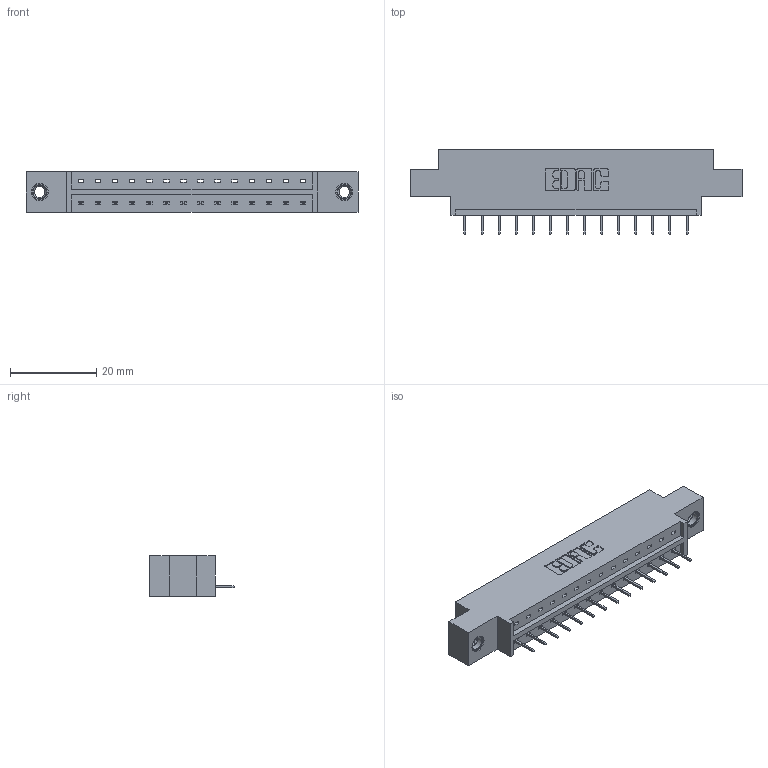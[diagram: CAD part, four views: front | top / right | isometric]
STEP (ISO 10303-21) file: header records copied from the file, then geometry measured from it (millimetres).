
FILE_DESCRIPTION (( 'STEP AP203' ), '1' );
FILE_NAME ('333-014-524-607.STEP', '2018-08-01T02:20:03', ( '' ), ( '' ), 'SwSTEP 2.0', 'SolidWorks 2016', '' );
FILE_SCHEMA (( 'CONFIG_CONTROL_DESIGN' ));
Length unit declared in the file: inch
Products named in the file (4): 333 Part_Offset - .156 Dia - TI; 345-292-001_345-293-124; 345-250-001_345-250-005-103; 333-014-524-607
Assembly tree (17 placements, depth 2):
  333-014-524-607
    333 Part_Offset - .156 Dia - TI
    345-292-001_345-293-124  x14
    345-250-001_345-250-005-103  x2
Bounding box: 77.01 x 19.69 x 9.4 mm (x, y, z)
Volume: 7212.2 mm3; surface area: 7665.7 mm2
Topology: 17 solids, 17 shells, 1046 faces, 2979 edges, 1922 vertices
Faces by surface type: plane 778, cylinder 252, cone 12, torus 4
Entity records: 13572 total; most frequent: CARTESIAN_POINT 2327, ORIENTED_EDGE 2270, DIRECTION 2053, EDGE_CURVE 1135, VECTOR 991, LINE 991, VERTEX_POINT 748, AXIS2_PLACEMENT_3D 531
